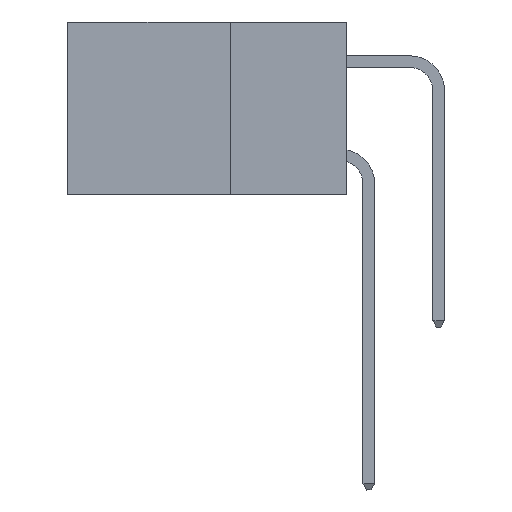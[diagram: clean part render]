
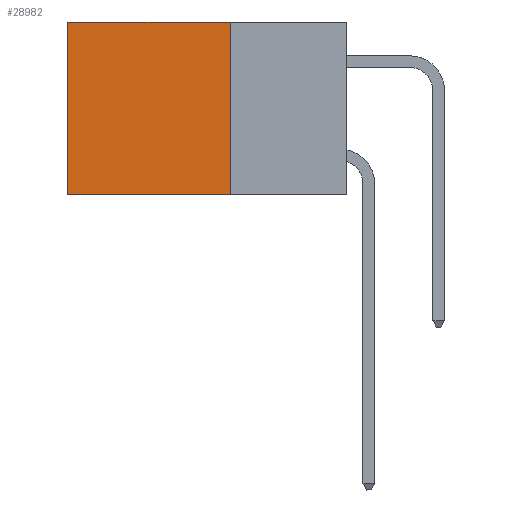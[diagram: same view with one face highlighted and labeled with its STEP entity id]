
A CAD part, left-side view. The second image highlights one B-rep face of the part: STEP entity #28982.
In plain terms, the highlighted planar face has unit normal (-1, 0, 0).
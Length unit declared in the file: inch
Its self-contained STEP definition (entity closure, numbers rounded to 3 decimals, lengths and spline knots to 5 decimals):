
#1210 = LINE ( 'NONE', #7708, #25830 ) ;
#2791 = ORIENTED_EDGE ( 'NONE', *, *, #7003, .F. ) ;
#2979 = CARTESIAN_POINT ( 'NONE',  ( 0.2875, 0.25, -0.37 ) ) ;
#3149 = CARTESIAN_POINT ( 'NONE',  ( 0.2875, 0.6, -0.37 ) ) ;
#3798 = PLANE ( 'NONE',  #40208 ) ;
#5942 = CARTESIAN_POINT ( 'NONE',  ( 0.2875, 0.25, -0.37 ) ) ;
#6094 = LINE ( 'NONE', #28913, #22225 ) ;
#7003 = EDGE_CURVE ( 'NONE', #19759, #17878, #24382, .T. ) ;
#7109 = CARTESIAN_POINT ( 'NONE',  ( 0.2875, 0.25, 0. ) ) ;
#7708 = CARTESIAN_POINT ( 'NONE',  ( 0.2875, 0.6, 0. ) ) ;
#8302 = ORIENTED_EDGE ( 'NONE', *, *, #30353, .T. ) ;
#10008 = DIRECTION ( 'NONE',  ( 0., 1., 0. ) ) ;
#10540 = DIRECTION ( 'NONE',  ( 1., 0., 0. ) ) ;
#10951 = FACE_OUTER_BOUND ( 'NONE', #18995, .T. ) ;
#11614 = DIRECTION ( 'NONE',  ( 0., 0., -1. ) ) ;
#14099 = DIRECTION ( 'NONE',  ( 0., 0., -1. ) ) ;
#17665 = VECTOR ( 'NONE', #10008, 39.37008 ) ;
#17878 = VERTEX_POINT ( 'NONE', #3149 ) ;
#18876 = EDGE_CURVE ( 'NONE', #24822, #19759, #6094, .T. ) ;
#18995 = EDGE_LOOP ( 'NONE', ( #40900, #2791, #32524, #8302 ) ) ;
#19759 = VERTEX_POINT ( 'NONE', #2979 ) ;
#22168 = DIRECTION ( 'NONE',  ( 0., 0., -1. ) ) ;
#22225 = VECTOR ( 'NONE', #11614, 39.37008 ) ;
#24382 = LINE ( 'NONE', #5942, #17665 ) ;
#24822 = VERTEX_POINT ( 'NONE', #45294 ) ;
#25830 = VECTOR ( 'NONE', #22168, 39.37008 ) ;
#28913 = CARTESIAN_POINT ( 'NONE',  ( 0.2875, 0.25, 0. ) ) ;
#28982 = ADVANCED_FACE ( 'NONE', ( #10951 ), #3798, .F. ) ;
#30353 = EDGE_CURVE ( 'NONE', #24822, #37447, #36561, .T. ) ;
#30789 = CARTESIAN_POINT ( 'NONE',  ( 0.2875, 0.6, 0. ) ) ;
#32524 = ORIENTED_EDGE ( 'NONE', *, *, #18876, .F. ) ;
#33498 = EDGE_CURVE ( 'NONE', #37447, #17878, #1210, .T. ) ;
#36561 = LINE ( 'NONE', #40077, #37154 ) ;
#37154 = VECTOR ( 'NONE', #39470, 39.37008 ) ;
#37447 = VERTEX_POINT ( 'NONE', #30789 ) ;
#39470 = DIRECTION ( 'NONE',  ( 0., 1., 0. ) ) ;
#40077 = CARTESIAN_POINT ( 'NONE',  ( 0.2875, 0.25, 0. ) ) ;
#40208 = AXIS2_PLACEMENT_3D ( 'NONE', #7109, #10540, #14099 ) ;
#40900 = ORIENTED_EDGE ( 'NONE', *, *, #33498, .T. ) ;
#45294 = CARTESIAN_POINT ( 'NONE',  ( 0.2875, 0.25, 0. ) ) ;
